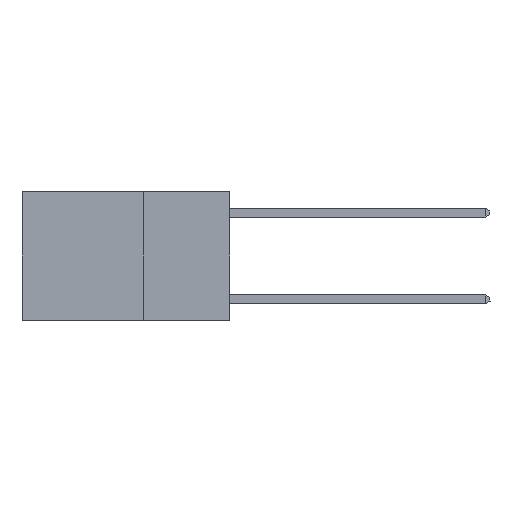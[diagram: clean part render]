
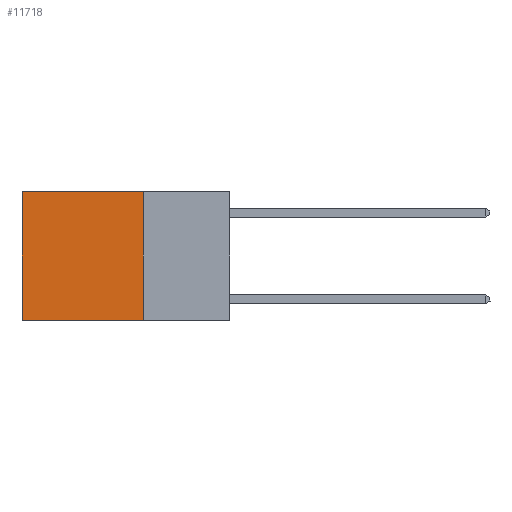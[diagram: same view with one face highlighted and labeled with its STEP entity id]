
A CAD part, left-side view. The second image highlights one B-rep face of the part: STEP entity #11718.
In plain terms, the highlighted planar face has unit normal (-1, 0, 0).
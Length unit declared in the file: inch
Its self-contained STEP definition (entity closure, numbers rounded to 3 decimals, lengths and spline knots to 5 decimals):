
#363 = ORIENTED_EDGE ( 'NONE', *, *, #4811, .T. ) ;
#410 = DIRECTION ( 'NONE',  ( 1., 0., 0. ) ) ;
#749 = EDGE_LOOP ( 'NONE', ( #363, #8640, #9989, #11097 ) ) ;
#1055 = AXIS2_PLACEMENT_3D ( 'NONE', #1523, #410, #8227 ) ;
#1383 = DIRECTION ( 'NONE',  ( 0., 1., 0. ) ) ;
#1510 = VERTEX_POINT ( 'NONE', #2541 ) ;
#1523 = CARTESIAN_POINT ( 'NONE',  ( 0.2625, 0.25, 0. ) ) ;
#2357 = CARTESIAN_POINT ( 'NONE',  ( 0.2625, 0.6, -0.37 ) ) ;
#2402 = VECTOR ( 'NONE', #7582, 39.37008 ) ;
#2541 = CARTESIAN_POINT ( 'NONE',  ( 0.2625, 0.6, 0. ) ) ;
#3205 = CARTESIAN_POINT ( 'NONE',  ( 0.2625, 0.6, 0. ) ) ;
#3673 = CARTESIAN_POINT ( 'NONE',  ( 0.2625, 0.25, -0.37 ) ) ;
#4811 = EDGE_CURVE ( 'NONE', #1510, #10265, #14045, .T. ) ;
#5060 = VECTOR ( 'NONE', #1383, 39.37008 ) ;
#5633 = EDGE_CURVE ( 'NONE', #6311, #10265, #7942, .T. ) ;
#6311 = VERTEX_POINT ( 'NONE', #3673 ) ;
#6519 = CARTESIAN_POINT ( 'NONE',  ( 0.2625, 0.25, 0. ) ) ;
#7160 = PLANE ( 'NONE',  #1055 ) ;
#7476 = CARTESIAN_POINT ( 'NONE',  ( 0.2625, 0.25, 0. ) ) ;
#7582 = DIRECTION ( 'NONE',  ( 0., 1., 0. ) ) ;
#7942 = LINE ( 'NONE', #8055, #5060 ) ;
#8055 = CARTESIAN_POINT ( 'NONE',  ( 0.2625, 0.25, -0.37 ) ) ;
#8090 = FACE_OUTER_BOUND ( 'NONE', #749, .T. ) ;
#8227 = DIRECTION ( 'NONE',  ( 0., 0., -1. ) ) ;
#8640 = ORIENTED_EDGE ( 'NONE', *, *, #5633, .F. ) ;
#9697 = DIRECTION ( 'NONE',  ( 0., 0., -1. ) ) ;
#9936 = CARTESIAN_POINT ( 'NONE',  ( 0.2625, 0.25, 0. ) ) ;
#9989 = ORIENTED_EDGE ( 'NONE', *, *, #11468, .F. ) ;
#10117 = VECTOR ( 'NONE', #11015, 39.37008 ) ;
#10265 = VERTEX_POINT ( 'NONE', #2357 ) ;
#10467 = LINE ( 'NONE', #9936, #10117 ) ;
#10758 = LINE ( 'NONE', #6519, #2402 ) ;
#11015 = DIRECTION ( 'NONE',  ( 0., 0., -1. ) ) ;
#11097 = ORIENTED_EDGE ( 'NONE', *, *, #11974, .T. ) ;
#11468 = EDGE_CURVE ( 'NONE', #12638, #6311, #10467, .T. ) ;
#11718 = ADVANCED_FACE ( 'NONE', ( #8090 ), #7160, .F. ) ;
#11974 = EDGE_CURVE ( 'NONE', #12638, #1510, #10758, .T. ) ;
#12638 = VERTEX_POINT ( 'NONE', #7476 ) ;
#13738 = VECTOR ( 'NONE', #9697, 39.37008 ) ;
#14045 = LINE ( 'NONE', #3205, #13738 ) ;
